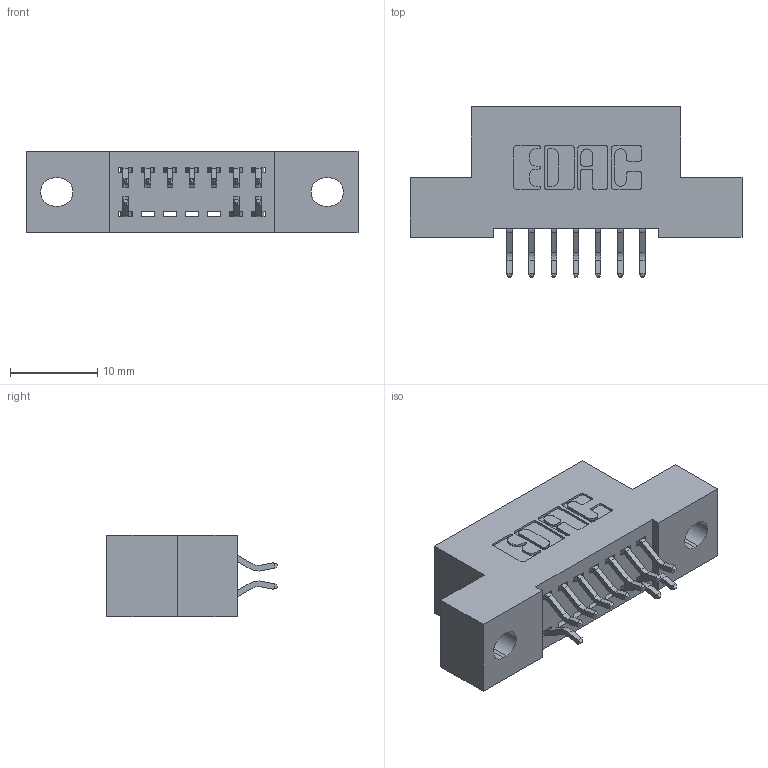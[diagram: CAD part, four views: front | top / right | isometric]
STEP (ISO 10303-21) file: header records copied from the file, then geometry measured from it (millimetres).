
FILE_DESCRIPTION (( 'STEP AP203' ), '1' );
FILE_NAME ('392-014-556-202.STEP', '2018-08-15T00:20:32', ( '' ), ( '' ), 'SwSTEP 2.0', 'SolidWorks 2016', '' );
FILE_SCHEMA (( 'CONFIG_CONTROL_DESIGN' ));
Length unit declared in the file: inch
Products named in the file (3): 342 Part_.128 Slot; 345-292-001_556 Tail; 392-014-556-202
Assembly tree (11 placements, depth 2):
  392-014-556-202
    342 Part_.128 Slot
    345-292-001_556 Tail  x10
Bounding box: 38.1 x 19.58 x 9.4 mm (x, y, z)
Volume: 3169.2 mm3; surface area: 3847.1 mm2
Topology: 11 solids, 11 shells, 718 faces, 2125 edges, 1402 vertices
Faces by surface type: plane 494, cylinder 224
Entity records: 9125 total; most frequent: CARTESIAN_POINT 1586, ORIENTED_EDGE 1514, DIRECTION 1401, EDGE_CURVE 757, LINE 621, VECTOR 621, VERTEX_POINT 502, AXIS2_PLACEMENT_3D 390
